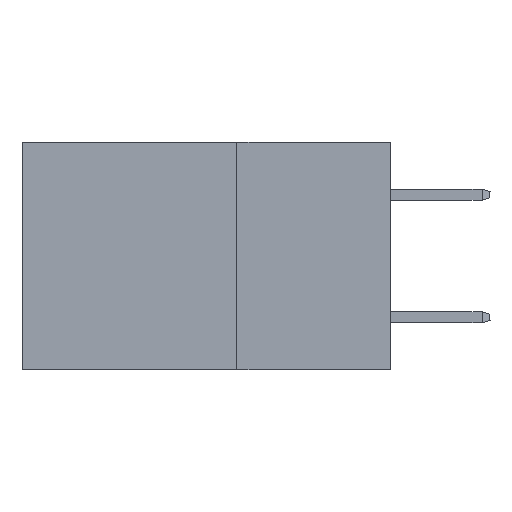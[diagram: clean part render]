
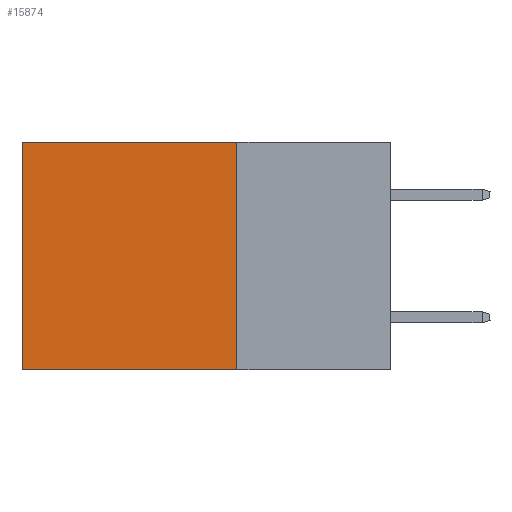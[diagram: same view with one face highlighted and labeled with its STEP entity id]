
A CAD part, left-side view. The second image highlights one B-rep face of the part: STEP entity #15874.
In plain terms, the highlighted planar face has unit normal (-1, 0, 0).
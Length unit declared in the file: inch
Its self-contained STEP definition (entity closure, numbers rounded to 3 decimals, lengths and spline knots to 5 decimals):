
#686 = VERTEX_POINT ( 'NONE', #7301 ) ;
#2508 = DIRECTION ( 'NONE',  ( 0., 0., -1. ) ) ;
#2583 = LINE ( 'NONE', #22342, #8217 ) ;
#4208 = FACE_OUTER_BOUND ( 'NONE', #14353, .T. ) ;
#6022 = EDGE_CURVE ( 'NONE', #8511, #686, #22827, .T. ) ;
#6297 = EDGE_CURVE ( 'NONE', #19939, #6920, #2583, .T. ) ;
#6838 = VECTOR ( 'NONE', #17190, 39.37008 ) ;
#6920 = VERTEX_POINT ( 'NONE', #19066 ) ;
#7301 = CARTESIAN_POINT ( 'NONE',  ( 0.2875, 0.6, -0.37 ) ) ;
#7601 = ORIENTED_EDGE ( 'NONE', *, *, #6022, .T. ) ;
#7646 = VECTOR ( 'NONE', #12714, 39.37008 ) ;
#8217 = VECTOR ( 'NONE', #2508, 39.37008 ) ;
#8511 = VERTEX_POINT ( 'NONE', #10984 ) ;
#10984 = CARTESIAN_POINT ( 'NONE',  ( 0.2875, 0.6, 0. ) ) ;
#11208 = ORIENTED_EDGE ( 'NONE', *, *, #13666, .T. ) ;
#11225 = CARTESIAN_POINT ( 'NONE',  ( 0.2875, 0.25, -0.37 ) ) ;
#12267 = CARTESIAN_POINT ( 'NONE',  ( 0.2875, 0.25, 0. ) ) ;
#12714 = DIRECTION ( 'NONE',  ( 0., 1., 0. ) ) ;
#13666 = EDGE_CURVE ( 'NONE', #19939, #8511, #22901, .T. ) ;
#13781 = DIRECTION ( 'NONE',  ( 0., 0., -1. ) ) ;
#14088 = DIRECTION ( 'NONE',  ( 0., 0., -1. ) ) ;
#14353 = EDGE_LOOP ( 'NONE', ( #7601, #20825, #19371, #11208 ) ) ;
#14872 = CARTESIAN_POINT ( 'NONE',  ( 0.2875, 0.25, 0. ) ) ;
#15072 = AXIS2_PLACEMENT_3D ( 'NONE', #12267, #20068, #14088 ) ;
#15874 = ADVANCED_FACE ( 'NONE', ( #4208 ), #24271, .F. ) ;
#16113 = CARTESIAN_POINT ( 'NONE',  ( 0.2875, 0.25, 0. ) ) ;
#17190 = DIRECTION ( 'NONE',  ( 0., 1., 0. ) ) ;
#19066 = CARTESIAN_POINT ( 'NONE',  ( 0.2875, 0.25, -0.37 ) ) ;
#19174 = EDGE_CURVE ( 'NONE', #6920, #686, #24572, .T. ) ;
#19371 = ORIENTED_EDGE ( 'NONE', *, *, #6297, .F. ) ;
#19939 = VERTEX_POINT ( 'NONE', #16113 ) ;
#20068 = DIRECTION ( 'NONE',  ( 1., 0., 0. ) ) ;
#20624 = VECTOR ( 'NONE', #13781, 39.37008 ) ;
#20825 = ORIENTED_EDGE ( 'NONE', *, *, #19174, .F. ) ;
#21865 = CARTESIAN_POINT ( 'NONE',  ( 0.2875, 0.6, 0. ) ) ;
#22342 = CARTESIAN_POINT ( 'NONE',  ( 0.2875, 0.25, 0. ) ) ;
#22827 = LINE ( 'NONE', #21865, #20624 ) ;
#22901 = LINE ( 'NONE', #14872, #7646 ) ;
#24271 = PLANE ( 'NONE',  #15072 ) ;
#24572 = LINE ( 'NONE', #11225, #6838 ) ;
